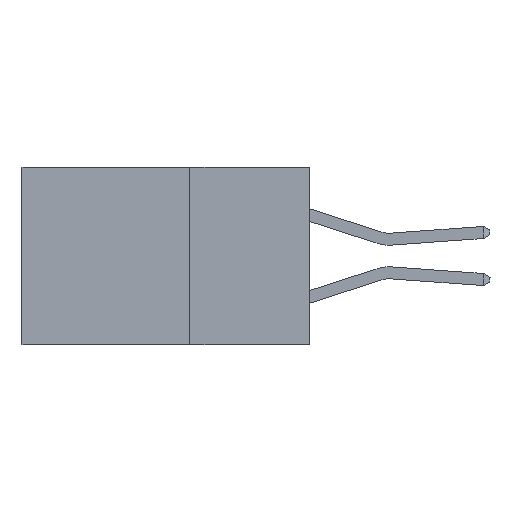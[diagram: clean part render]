
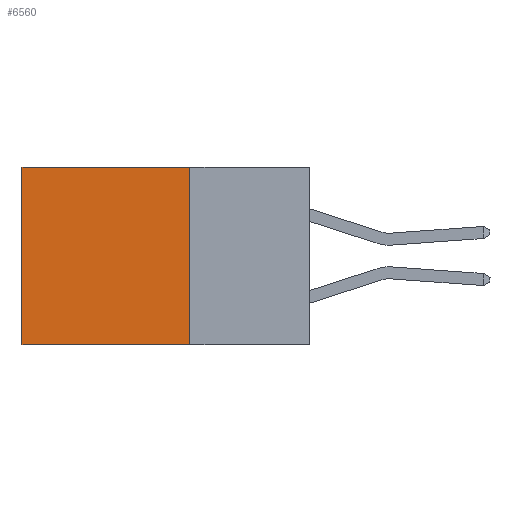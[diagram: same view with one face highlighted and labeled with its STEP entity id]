
A CAD part, left-side view. The second image highlights one B-rep face of the part: STEP entity #6560.
In plain terms, the highlighted planar face has unit normal (-1, 0, 0).
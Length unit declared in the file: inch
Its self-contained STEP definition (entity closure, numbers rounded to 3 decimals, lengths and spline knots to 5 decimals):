
#93 = ORIENTED_EDGE ( 'NONE', *, *, #10764, .T. ) ;
#852 = CARTESIAN_POINT ( 'NONE',  ( 0.298, 0.25, 0. ) ) ;
#1003 = CARTESIAN_POINT ( 'NONE',  ( 0.298, 0.6, 0. ) ) ;
#1736 = AXIS2_PLACEMENT_3D ( 'NONE', #6977, #12106, #4790 ) ;
#2131 = CARTESIAN_POINT ( 'NONE',  ( 0.298, 0.25, 0. ) ) ;
#2250 = CARTESIAN_POINT ( 'NONE',  ( 0.298, 0.6, 0. ) ) ;
#2953 = VERTEX_POINT ( 'NONE', #5251 ) ;
#3527 = LINE ( 'NONE', #2250, #13769 ) ;
#3752 = PLANE ( 'NONE',  #1736 ) ;
#4723 = EDGE_LOOP ( 'NONE', ( #9892, #8603, #13831, #93 ) ) ;
#4790 = DIRECTION ( 'NONE',  ( 0., 0., -1. ) ) ;
#5251 = CARTESIAN_POINT ( 'NONE',  ( 0.298, 0.25, 0. ) ) ;
#6268 = EDGE_CURVE ( 'NONE', #12526, #12976, #3527, .T. ) ;
#6560 = ADVANCED_FACE ( 'NONE', ( #13413 ), #3752, .F. ) ;
#6811 = DIRECTION ( 'NONE',  ( 0., 1., 0. ) ) ;
#6977 = CARTESIAN_POINT ( 'NONE',  ( 0.298, 0.25, 0. ) ) ;
#7303 = EDGE_CURVE ( 'NONE', #8346, #12976, #9593, .T. ) ;
#8286 = LINE ( 'NONE', #2131, #12790 ) ;
#8346 = VERTEX_POINT ( 'NONE', #12135 ) ;
#8603 = ORIENTED_EDGE ( 'NONE', *, *, #7303, .F. ) ;
#9593 = LINE ( 'NONE', #13192, #11064 ) ;
#9728 = EDGE_CURVE ( 'NONE', #2953, #8346, #10442, .T. ) ;
#9805 = DIRECTION ( 'NONE',  ( 0., 0., -1. ) ) ;
#9892 = ORIENTED_EDGE ( 'NONE', *, *, #6268, .T. ) ;
#9912 = CARTESIAN_POINT ( 'NONE',  ( 0.298, 0.6, -0.37 ) ) ;
#10442 = LINE ( 'NONE', #852, #10601 ) ;
#10601 = VECTOR ( 'NONE', #12509, 39.37008 ) ;
#10764 = EDGE_CURVE ( 'NONE', #2953, #12526, #8286, .T. ) ;
#11064 = VECTOR ( 'NONE', #6811, 39.37008 ) ;
#11625 = DIRECTION ( 'NONE',  ( 0., 1., 0. ) ) ;
#12106 = DIRECTION ( 'NONE',  ( 1., 0., 0. ) ) ;
#12135 = CARTESIAN_POINT ( 'NONE',  ( 0.298, 0.25, -0.37 ) ) ;
#12509 = DIRECTION ( 'NONE',  ( 0., 0., -1. ) ) ;
#12526 = VERTEX_POINT ( 'NONE', #1003 ) ;
#12790 = VECTOR ( 'NONE', #11625, 39.37008 ) ;
#12976 = VERTEX_POINT ( 'NONE', #9912 ) ;
#13192 = CARTESIAN_POINT ( 'NONE',  ( 0.298, 0.25, -0.37 ) ) ;
#13413 = FACE_OUTER_BOUND ( 'NONE', #4723, .T. ) ;
#13769 = VECTOR ( 'NONE', #9805, 39.37008 ) ;
#13831 = ORIENTED_EDGE ( 'NONE', *, *, #9728, .F. ) ;
